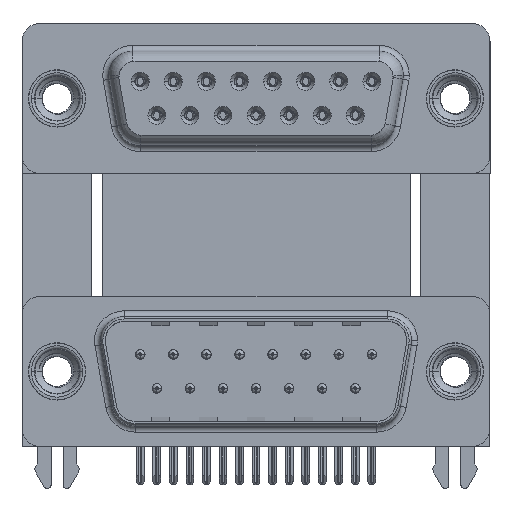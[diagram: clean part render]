
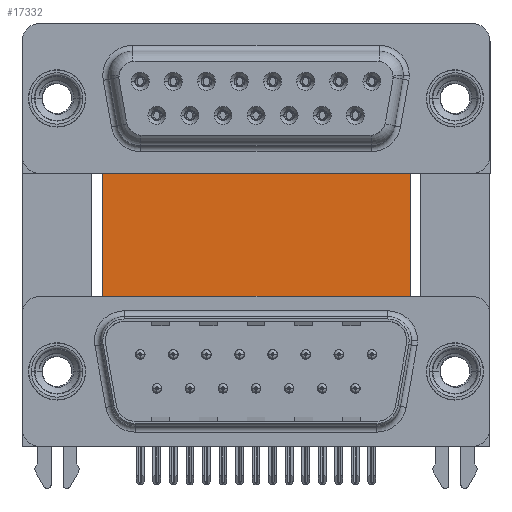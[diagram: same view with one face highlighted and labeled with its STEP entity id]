
A CAD part, top view. The second image highlights one B-rep face of the part: STEP entity #17332.
In plain terms, the highlighted planar face has unit normal (0, 0, 1).
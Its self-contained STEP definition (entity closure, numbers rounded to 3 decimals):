
#556 = VERTEX_POINT ( 'NONE', #36296 ) ;
#3380 = LINE ( 'NONE', #10784, #31079 ) ;
#3395 = DIRECTION ( 'NONE',  ( 1., 0., 0. ) ) ;
#5208 = VECTOR ( 'NONE', #40588, 1000. ) ;
#6872 = CARTESIAN_POINT ( 'NONE',  ( 3.79, -3.735, -12. ) ) ;
#8747 = PLANE ( 'NONE',  #36869 ) ;
#8786 = ORIENTED_EDGE ( 'NONE', *, *, #32728, .T. ) ;
#9126 = VERTEX_POINT ( 'NONE', #38328 ) ;
#10784 = CARTESIAN_POINT ( 'NONE',  ( 3.79, 16.585, -12. ) ) ;
#11671 = ORIENTED_EDGE ( 'NONE', *, *, #13470, .F. ) ;
#12033 = LINE ( 'NONE', #25721, #23039 ) ;
#13470 = EDGE_CURVE ( 'NONE', #13566, #556, #12033, .T. ) ;
#13566 = VERTEX_POINT ( 'NONE', #27339 ) ;
#17263 = VECTOR ( 'NONE', #3395, 1000. ) ;
#17304 = LINE ( 'NONE', #6872, #17263 ) ;
#17332 = ADVANCED_FACE ( 'NONE', ( #22041 ), #8747, .F. ) ;
#17840 = CARTESIAN_POINT ( 'NONE',  ( 3.79, 16.585, -12. ) ) ;
#18081 = EDGE_LOOP ( 'NONE', ( #33157, #24120, #11671, #8786 ) ) ;
#22041 = FACE_OUTER_BOUND ( 'NONE', #18081, .T. ) ;
#23039 = VECTOR ( 'NONE', #26190, 1000. ) ;
#23364 = VERTEX_POINT ( 'NONE', #37075 ) ;
#24120 = ORIENTED_EDGE ( 'NONE', *, *, #44516, .F. ) ;
#25519 = DIRECTION ( 'NONE',  ( -1., 0., 0. ) ) ;
#25721 = CARTESIAN_POINT ( 'NONE',  ( 3.79, 16.585, -12. ) ) ;
#26190 = DIRECTION ( 'NONE',  ( 1., 0., 0. ) ) ;
#27339 = CARTESIAN_POINT ( 'NONE',  ( 3.79, 16.585, -12. ) ) ;
#29244 = DIRECTION ( 'NONE',  ( 0., 0., -1. ) ) ;
#31079 = VECTOR ( 'NONE', #45675, 1000. ) ;
#32728 = EDGE_CURVE ( 'NONE', #13566, #9126, #3380, .T. ) ;
#33157 = ORIENTED_EDGE ( 'NONE', *, *, #41082, .T. ) ;
#36296 = CARTESIAN_POINT ( 'NONE',  ( 29.58, 16.585, -12. ) ) ;
#36869 = AXIS2_PLACEMENT_3D ( 'NONE', #17840, #29244, #25519 ) ;
#37075 = CARTESIAN_POINT ( 'NONE',  ( 29.58, -3.735, -12. ) ) ;
#38328 = CARTESIAN_POINT ( 'NONE',  ( 3.79, -3.735, -12. ) ) ;
#40588 = DIRECTION ( 'NONE',  ( 0., -1., 0. ) ) ;
#41082 = EDGE_CURVE ( 'NONE', #9126, #23364, #17304, .T. ) ;
#44081 = CARTESIAN_POINT ( 'NONE',  ( 29.58, 16.585, -12. ) ) ;
#44516 = EDGE_CURVE ( 'NONE', #556, #23364, #44533, .T. ) ;
#44533 = LINE ( 'NONE', #44081, #5208 ) ;
#45675 = DIRECTION ( 'NONE',  ( 0., -1., 0. ) ) ;
